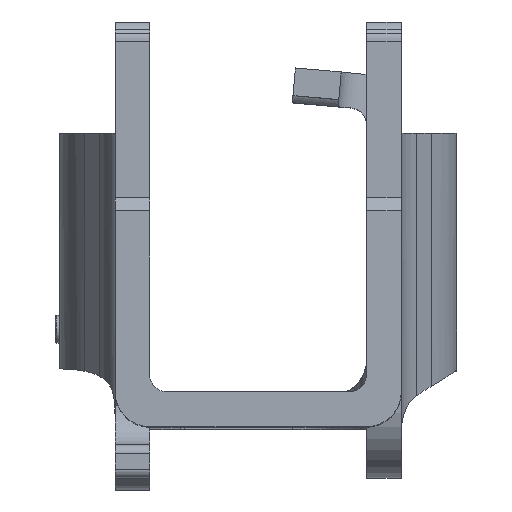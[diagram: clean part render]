
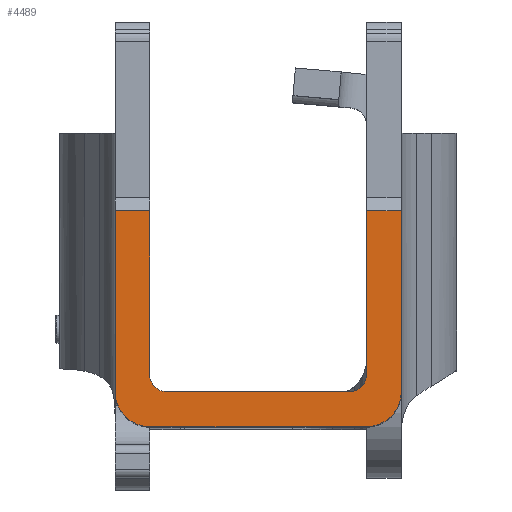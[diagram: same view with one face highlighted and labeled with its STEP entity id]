
A CAD part, top view. The second image highlights one B-rep face of the part: STEP entity #4489.
In plain terms, the highlighted planar face has unit normal (0, 0, 1).
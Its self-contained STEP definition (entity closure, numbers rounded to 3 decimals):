
#211=PLANE('',#4940);
#437=FACE_OUTER_BOUND('',#673,.T.);
#673=EDGE_LOOP('',(#4148,#4149,#4150,#4151,#4152,#4153,#4154,#4155,#4156,
#4157,#4158,#4159));
#698=LINE('',#6337,#1133);
#716=LINE('',#6398,#1151);
#730=LINE('',#6429,#1165);
#743=LINE('',#6464,#1178);
#995=LINE('',#7434,#1430);
#996=LINE('',#7436,#1431);
#1026=LINE('',#7543,#1461);
#1070=LINE('',#7680,#1505);
#1133=VECTOR('',#5011,10.);
#1151=VECTOR('',#5061,10.);
#1165=VECTOR('',#5087,10.);
#1178=VECTOR('',#5114,10.);
#1430=VECTOR('',#5864,10.);
#1431=VECTOR('',#5867,10.);
#1461=VECTOR('',#5967,10.);
#1505=VECTOR('',#6119,10.);
#1707=CIRCLE('',#4877,1.);
#1708=CIRCLE('',#4884,2.);
#1709=CIRCLE('',#4892,2.);
#1711=CIRCLE('',#4896,1.);
#1748=VERTEX_POINT('',#6334);
#1749=VERTEX_POINT('',#6336);
#1775=VERTEX_POINT('',#6395);
#1776=VERTEX_POINT('',#6397);
#1786=VERTEX_POINT('',#6426);
#1787=VERTEX_POINT('',#6428);
#1801=VERTEX_POINT('',#6461);
#1802=VERTEX_POINT('',#6463);
#2129=VERTEX_POINT('',#7539);
#2131=VERTEX_POINT('',#7542);
#2153=VERTEX_POINT('',#7652);
#2154=VERTEX_POINT('',#7676);
#2195=EDGE_CURVE('',#1749,#1748,#698,.T.);
#2225=EDGE_CURVE('',#1776,#1775,#716,.T.);
#2241=EDGE_CURVE('',#1787,#1786,#730,.T.);
#2259=EDGE_CURVE('',#1802,#1801,#743,.T.);
#2674=EDGE_CURVE('',#1801,#1776,#995,.T.);
#2675=EDGE_CURVE('',#1786,#1749,#996,.T.);
#2719=EDGE_CURVE('',#2131,#2129,#1026,.T.);
#2770=EDGE_CURVE('',#2131,#1748,#1707,.T.);
#2775=EDGE_CURVE('',#2153,#1775,#1708,.T.);
#2780=EDGE_CURVE('',#1787,#2154,#1709,.T.);
#2782=EDGE_CURVE('',#2153,#2154,#1070,.T.);
#2784=EDGE_CURVE('',#1802,#2129,#1711,.T.);
#4148=ORIENTED_EDGE('',*,*,#2675,.T.);
#4149=ORIENTED_EDGE('',*,*,#2195,.T.);
#4150=ORIENTED_EDGE('',*,*,#2770,.F.);
#4151=ORIENTED_EDGE('',*,*,#2719,.T.);
#4152=ORIENTED_EDGE('',*,*,#2784,.F.);
#4153=ORIENTED_EDGE('',*,*,#2259,.T.);
#4154=ORIENTED_EDGE('',*,*,#2674,.T.);
#4155=ORIENTED_EDGE('',*,*,#2225,.T.);
#4156=ORIENTED_EDGE('',*,*,#2775,.F.);
#4157=ORIENTED_EDGE('',*,*,#2782,.T.);
#4158=ORIENTED_EDGE('',*,*,#2780,.F.);
#4159=ORIENTED_EDGE('',*,*,#2241,.T.);
#4489=ADVANCED_FACE('',(#437),#211,.T.);
#4877=AXIS2_PLACEMENT_3D('',#7642,#6078,#6079);
#4884=AXIS2_PLACEMENT_3D('',#7654,#6096,#6097);
#4892=AXIS2_PLACEMENT_3D('',#7677,#6114,#6115);
#4896=AXIS2_PLACEMENT_3D('',#7684,#6124,#6125);
#4940=AXIS2_PLACEMENT_3D('',#7766,#6250,#6251);
#5011=DIRECTION('',(0.,-1.,0.));
#5061=DIRECTION('',(0.,-1.,0.));
#5087=DIRECTION('',(0.,1.,0.));
#5114=DIRECTION('',(0.,1.,0.));
#5864=DIRECTION('',(-1.,0.,0.));
#5867=DIRECTION('',(-1.,0.,0.));
#5967=DIRECTION('',(-1.,0.,0.));
#6078=DIRECTION('center_axis',(0.,0.,1.));
#6079=DIRECTION('ref_axis',(0.707,-0.707,0.));
#6096=DIRECTION('center_axis',(0.,0.,-1.));
#6097=DIRECTION('ref_axis',(-0.707,-0.707,0.));
#6114=DIRECTION('center_axis',(0.,0.,-1.));
#6115=DIRECTION('ref_axis',(0.707,-0.707,0.));
#6119=DIRECTION('',(1.,0.,0.));
#6124=DIRECTION('center_axis',(0.,0.,1.));
#6125=DIRECTION('ref_axis',(-0.707,-0.707,0.));
#6250=DIRECTION('center_axis',(0.,0.,1.));
#6251=DIRECTION('ref_axis',(1.,0.,0.));
#6334=CARTESIAN_POINT('',(6.25,-15.8,110.25));
#6336=CARTESIAN_POINT('',(6.25,-6.36,110.25));
#6337=CARTESIAN_POINT('',(6.25,-1.81,110.25));
#6395=CARTESIAN_POINT('',(-8.25,-16.8,110.25));
#6397=CARTESIAN_POINT('',(-8.25,-6.36,110.25));
#6398=CARTESIAN_POINT('',(-8.25,-1.81,110.25));
#6426=CARTESIAN_POINT('',(8.25,-6.36,110.25));
#6428=CARTESIAN_POINT('',(8.25,-16.8,110.25));
#6429=CARTESIAN_POINT('',(8.25,-18.8,110.25));
#6461=CARTESIAN_POINT('',(-6.25,-6.36,110.25));
#6463=CARTESIAN_POINT('',(-6.25,-15.8,110.25));
#6464=CARTESIAN_POINT('',(-6.25,-16.8,110.25));
#7434=CARTESIAN_POINT('',(4.125,-6.36,110.25));
#7436=CARTESIAN_POINT('',(4.125,-6.36,110.25));
#7539=CARTESIAN_POINT('',(-5.25,-16.8,110.25));
#7542=CARTESIAN_POINT('',(5.25,-16.8,110.25));
#7543=CARTESIAN_POINT('',(6.25,-16.8,110.25));
#7642=CARTESIAN_POINT('Origin',(5.25,-15.8,110.25));
#7652=CARTESIAN_POINT('',(-6.25,-18.8,110.25));
#7654=CARTESIAN_POINT('Origin',(-6.25,-16.8,110.25));
#7676=CARTESIAN_POINT('',(6.25,-18.8,110.25));
#7677=CARTESIAN_POINT('Origin',(6.25,-16.8,110.25));
#7680=CARTESIAN_POINT('',(-8.25,-18.8,110.25));
#7684=CARTESIAN_POINT('Origin',(-5.25,-15.8,110.25));
#7766=CARTESIAN_POINT('Origin',(0.,-10.305,110.25));
